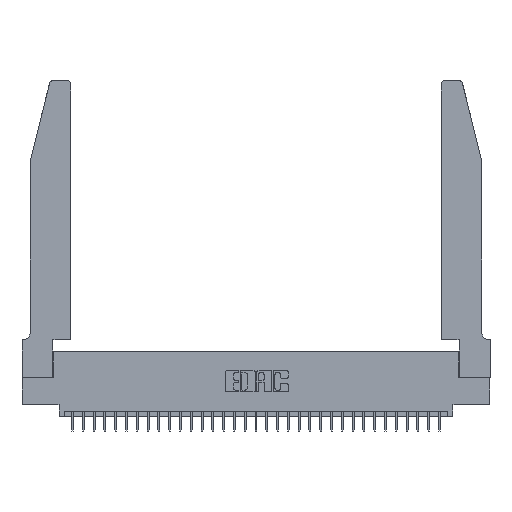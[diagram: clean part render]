
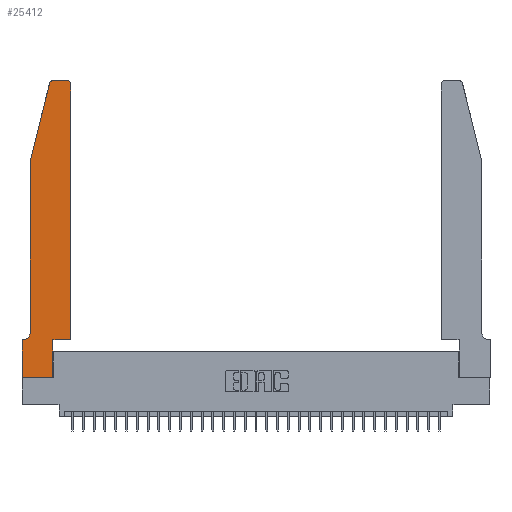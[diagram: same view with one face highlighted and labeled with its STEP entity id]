
A CAD part, top view. The second image highlights one B-rep face of the part: STEP entity #25412.
In plain terms, the highlighted planar face has unit normal (0, 0, 1).
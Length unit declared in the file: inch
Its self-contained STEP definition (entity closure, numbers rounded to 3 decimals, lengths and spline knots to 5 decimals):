
#127 = AXIS2_PLACEMENT_3D ( 'NONE', #167, #5073, #25361 ) ;
#167 = CARTESIAN_POINT ( 'NONE',  ( 0.0055, 0.42, 0.37 ) ) ;
#191 = ORIENTED_EDGE ( 'NONE', *, *, #1535, .T. ) ;
#290 = LINE ( 'NONE', #23934, #26153 ) ;
#510 = AXIS2_PLACEMENT_3D ( 'NONE', #31158, #7992, #17622 ) ;
#616 = VERTEX_POINT ( 'NONE', #8113 ) ;
#1226 = LINE ( 'NONE', #31824, #9081 ) ;
#1312 = EDGE_CURVE ( 'NONE', #24354, #18699, #17097, .T. ) ;
#1509 = VERTEX_POINT ( 'NONE', #23009 ) ;
#1535 = EDGE_CURVE ( 'NONE', #18699, #32676, #20452, .T. ) ;
#1773 = DIRECTION ( 'NONE',  ( -0.239, -0.971, 0. ) ) ;
#2250 = VECTOR ( 'NONE', #31220, 39.37008 ) ;
#2368 = ORIENTED_EDGE ( 'NONE', *, *, #1312, .T. ) ;
#2756 = EDGE_LOOP ( 'NONE', ( #27549, #12224, #2368, #191, #10371, #13949, #21855, #21083, #14278, #10070, #6058, #8004 ) ) ;
#2759 = CARTESIAN_POINT ( 'NONE',  ( 0.0755, 2., 0.37 ) ) ;
#3053 = EDGE_CURVE ( 'NONE', #616, #24354, #28037, .T. ) ;
#3518 = DIRECTION ( 'NONE',  ( 0., 1., 0. ) ) ;
#3597 = CARTESIAN_POINT ( 'NONE',  ( 0., 0.35, 0.37 ) ) ;
#3937 = CIRCLE ( 'NONE', #11415, 0.03 ) ;
#5073 = DIRECTION ( 'NONE',  ( 0., 0., -1. ) ) ;
#5215 = CARTESIAN_POINT ( 'NONE',  ( 0.2865, 0.35, 0.37 ) ) ;
#6058 = ORIENTED_EDGE ( 'NONE', *, *, #28293, .T. ) ;
#6109 = FACE_OUTER_BOUND ( 'NONE', #2756, .T. ) ;
#6496 = CARTESIAN_POINT ( 'NONE',  ( 0.4505, 0.35, 0.37 ) ) ;
#6671 = DIRECTION ( 'NONE',  ( 1., 0., 0. ) ) ;
#6859 = VERTEX_POINT ( 'NONE', #23536 ) ;
#6990 = CARTESIAN_POINT ( 'NONE',  ( 0.0755, 2., 0.37 ) ) ;
#7638 = DIRECTION ( 'NONE',  ( 0., -1., 0. ) ) ;
#7777 = CARTESIAN_POINT ( 'NONE',  ( 0.4205, 2.75, 0.37 ) ) ;
#7885 = DIRECTION ( 'NONE',  ( 1., 0., 0. ) ) ;
#7992 = DIRECTION ( 'NONE',  ( 0., 0., 1. ) ) ;
#8004 = ORIENTED_EDGE ( 'NONE', *, *, #23946, .T. ) ;
#8113 = CARTESIAN_POINT ( 'NONE',  ( 0.284, 2.75, 0.37 ) ) ;
#8885 = CARTESIAN_POINT ( 'NONE',  ( 0.0755, 0.42, 0.37 ) ) ;
#9081 = VECTOR ( 'NONE', #31985, 39.37008 ) ;
#9664 = CARTESIAN_POINT ( 'NONE',  ( 0.4205, 2.72, 0.37 ) ) ;
#10070 = ORIENTED_EDGE ( 'NONE', *, *, #22429, .T. ) ;
#10371 = ORIENTED_EDGE ( 'NONE', *, *, #20257, .T. ) ;
#10435 = CARTESIAN_POINT ( 'NONE',  ( 0.4505, 2.72, 0.37 ) ) ;
#10689 = VERTEX_POINT ( 'NONE', #22697 ) ;
#11415 = AXIS2_PLACEMENT_3D ( 'NONE', #9664, #20132, #12519 ) ;
#11919 = LINE ( 'NONE', #22933, #2250 ) ;
#12004 = LINE ( 'NONE', #6496, #26129 ) ;
#12116 = VERTEX_POINT ( 'NONE', #10435 ) ;
#12224 = ORIENTED_EDGE ( 'NONE', *, *, #3053, .T. ) ;
#12519 = DIRECTION ( 'NONE',  ( 1., 0., 0. ) ) ;
#12790 = VECTOR ( 'NONE', #1773, 39.37008 ) ;
#13325 = EDGE_CURVE ( 'NONE', #10689, #1509, #15799, .T. ) ;
#13654 = EDGE_CURVE ( 'NONE', #28058, #616, #1226, .T. ) ;
#13949 = ORIENTED_EDGE ( 'NONE', *, *, #22705, .T. ) ;
#14278 = ORIENTED_EDGE ( 'NONE', *, *, #20870, .T. ) ;
#14509 = PLANE ( 'NONE',  #29829 ) ;
#14527 = VERTEX_POINT ( 'NONE', #27911 ) ;
#15500 = VERTEX_POINT ( 'NONE', #27758 ) ;
#15799 = LINE ( 'NONE', #24100, #17151 ) ;
#15874 = LINE ( 'NONE', #18391, #33181 ) ;
#16969 = CARTESIAN_POINT ( 'NONE',  ( 0.2865, 0.35, 0.37 ) ) ;
#16979 = CARTESIAN_POINT ( 'NONE',  ( 0.0755, 2., 0.37 ) ) ;
#17097 = LINE ( 'NONE', #6990, #12790 ) ;
#17151 = VECTOR ( 'NONE', #7885, 39.37008 ) ;
#17622 = DIRECTION ( 'NONE',  ( 1., 0., 0. ) ) ;
#18309 = EDGE_CURVE ( 'NONE', #6859, #10689, #11919, .T. ) ;
#18332 = VERTEX_POINT ( 'NONE', #5215 ) ;
#18391 = CARTESIAN_POINT ( 'NONE',  ( 0.0755, 0.35, 0.37 ) ) ;
#18699 = VERTEX_POINT ( 'NONE', #16979 ) ;
#18718 = VECTOR ( 'NONE', #7638, 39.37008 ) ;
#19245 = DIRECTION ( 'NONE',  ( 0., 0., 1. ) ) ;
#19650 = LINE ( 'NONE', #16969, #22800 ) ;
#20132 = DIRECTION ( 'NONE',  ( 0., 0., 1. ) ) ;
#20257 = EDGE_CURVE ( 'NONE', #32676, #14527, #20576, .T. ) ;
#20452 = LINE ( 'NONE', #2759, #18718 ) ;
#20576 = CIRCLE ( 'NONE', #127, 0.07 ) ;
#20870 = EDGE_CURVE ( 'NONE', #1509, #18332, #19650, .T. ) ;
#21083 = ORIENTED_EDGE ( 'NONE', *, *, #13325, .T. ) ;
#21855 = ORIENTED_EDGE ( 'NONE', *, *, #18309, .T. ) ;
#22429 = EDGE_CURVE ( 'NONE', #18332, #15500, #12004, .T. ) ;
#22697 = CARTESIAN_POINT ( 'NONE',  ( 0., 0., 0.37 ) ) ;
#22705 = EDGE_CURVE ( 'NONE', #14527, #6859, #15874, .T. ) ;
#22800 = VECTOR ( 'NONE', #32233, 39.37008 ) ;
#22933 = CARTESIAN_POINT ( 'NONE',  ( 0., 0., 0.37 ) ) ;
#23009 = CARTESIAN_POINT ( 'NONE',  ( 0.2865, 0., 0.37 ) ) ;
#23536 = CARTESIAN_POINT ( 'NONE',  ( 0., 0.35, 0.37 ) ) ;
#23926 = CARTESIAN_POINT ( 'NONE',  ( 0.25487, 2.72718, 0.37 ) ) ;
#23934 = CARTESIAN_POINT ( 'NONE',  ( 0.4505, 0.35, 0.37 ) ) ;
#23946 = EDGE_CURVE ( 'NONE', #12116, #28058, #3937, .T. ) ;
#24100 = CARTESIAN_POINT ( 'NONE',  ( 0., 0., 0.37 ) ) ;
#24354 = VERTEX_POINT ( 'NONE', #23926 ) ;
#24358 = DIRECTION ( 'NONE',  ( 1., 0., 0. ) ) ;
#25361 = DIRECTION ( 'NONE',  ( -1., 0., 0. ) ) ;
#25412 = ADVANCED_FACE ( 'NONE', ( #6109 ), #14509, .T. ) ;
#26077 = DIRECTION ( 'NONE',  ( -1., 0., 0. ) ) ;
#26129 = VECTOR ( 'NONE', #6671, 39.37008 ) ;
#26153 = VECTOR ( 'NONE', #3518, 39.37008 ) ;
#27549 = ORIENTED_EDGE ( 'NONE', *, *, #13654, .T. ) ;
#27758 = CARTESIAN_POINT ( 'NONE',  ( 0.4505, 0.35, 0.37 ) ) ;
#27911 = CARTESIAN_POINT ( 'NONE',  ( 0.0055, 0.35, 0.37 ) ) ;
#28037 = CIRCLE ( 'NONE', #510, 0.03 ) ;
#28058 = VERTEX_POINT ( 'NONE', #7777 ) ;
#28293 = EDGE_CURVE ( 'NONE', #15500, #12116, #290, .T. ) ;
#29829 = AXIS2_PLACEMENT_3D ( 'NONE', #3597, #19245, #24358 ) ;
#31158 = CARTESIAN_POINT ( 'NONE',  ( 0.284, 2.72, 0.37 ) ) ;
#31220 = DIRECTION ( 'NONE',  ( 0., -1., 0. ) ) ;
#31824 = CARTESIAN_POINT ( 'NONE',  ( 0.2605, 2.75, 0.37 ) ) ;
#31985 = DIRECTION ( 'NONE',  ( -1., 0., 0. ) ) ;
#32233 = DIRECTION ( 'NONE',  ( 0., 1., 0. ) ) ;
#32676 = VERTEX_POINT ( 'NONE', #8885 ) ;
#33181 = VECTOR ( 'NONE', #26077, 39.37008 ) ;
